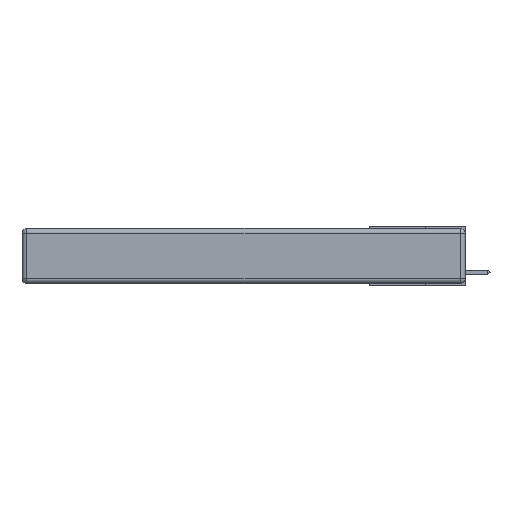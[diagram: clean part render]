
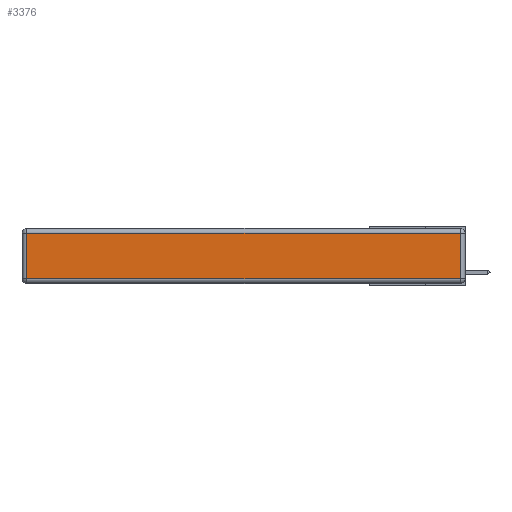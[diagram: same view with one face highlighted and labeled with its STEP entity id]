
A CAD part, left-side view. The second image highlights one B-rep face of the part: STEP entity #3376.
In plain terms, the highlighted planar face has unit normal (-1, 0, 0).
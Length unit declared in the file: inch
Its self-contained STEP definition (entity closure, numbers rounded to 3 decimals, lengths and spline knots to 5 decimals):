
#200 = CARTESIAN_POINT ( 'NONE',  ( 0., 0.03, -0.03 ) ) ;
#442 = DIRECTION ( 'NONE',  ( -1., 0., 0. ) ) ;
#705 = VECTOR ( 'NONE', #13233, 39.37008 ) ;
#1775 = EDGE_CURVE ( 'NONE', #12748, #6245, #12069, .T. ) ;
#3376 = ADVANCED_FACE ( 'NONE', ( #9781 ), #3655, .T. ) ;
#3609 = CARTESIAN_POINT ( 'NONE',  ( 0., 0., -0.343 ) ) ;
#3655 = PLANE ( 'NONE',  #8457 ) ;
#4084 = DIRECTION ( 'NONE',  ( 0., 0., -1. ) ) ;
#4110 = VERTEX_POINT ( 'NONE', #8952 ) ;
#4281 = VECTOR ( 'NONE', #13092, 39.37008 ) ;
#4509 = ORIENTED_EDGE ( 'NONE', *, *, #4553, .T. ) ;
#4553 = EDGE_CURVE ( 'NONE', #10756, #4110, #8349, .T. ) ;
#4689 = CARTESIAN_POINT ( 'NONE',  ( 0., 0.03, -0.343 ) ) ;
#5561 = EDGE_LOOP ( 'NONE', ( #4509, #13835, #14050, #12268 ) ) ;
#6245 = VERTEX_POINT ( 'NONE', #13334 ) ;
#6265 = CARTESIAN_POINT ( 'NONE',  ( 0., 2.72, -0.343 ) ) ;
#6548 = LINE ( 'NONE', #6265, #13124 ) ;
#6979 = DIRECTION ( 'NONE',  ( 0., 0., 1. ) ) ;
#7462 = VECTOR ( 'NONE', #6979, 39.37008 ) ;
#7512 = EDGE_CURVE ( 'NONE', #4110, #12748, #10045, .T. ) ;
#8291 = CARTESIAN_POINT ( 'NONE',  ( 0., 2.75, -0.03 ) ) ;
#8349 = LINE ( 'NONE', #11104, #705 ) ;
#8440 = CARTESIAN_POINT ( 'NONE',  ( 0., 2.72, -0.313 ) ) ;
#8457 = AXIS2_PLACEMENT_3D ( 'NONE', #3609, #442, #13680 ) ;
#8952 = CARTESIAN_POINT ( 'NONE',  ( 0., 0.03, -0.313 ) ) ;
#9441 = EDGE_CURVE ( 'NONE', #6245, #10756, #6548, .T. ) ;
#9781 = FACE_OUTER_BOUND ( 'NONE', #5561, .T. ) ;
#10045 = LINE ( 'NONE', #4689, #7462 ) ;
#10756 = VERTEX_POINT ( 'NONE', #8440 ) ;
#11104 = CARTESIAN_POINT ( 'NONE',  ( 0., 0., -0.313 ) ) ;
#12069 = LINE ( 'NONE', #8291, #4281 ) ;
#12268 = ORIENTED_EDGE ( 'NONE', *, *, #9441, .T. ) ;
#12748 = VERTEX_POINT ( 'NONE', #200 ) ;
#13092 = DIRECTION ( 'NONE',  ( 0., 1., 0. ) ) ;
#13124 = VECTOR ( 'NONE', #4084, 39.37008 ) ;
#13233 = DIRECTION ( 'NONE',  ( 0., -1., 0. ) ) ;
#13334 = CARTESIAN_POINT ( 'NONE',  ( 0., 2.72, -0.03 ) ) ;
#13680 = DIRECTION ( 'NONE',  ( 0., 0., 1. ) ) ;
#13835 = ORIENTED_EDGE ( 'NONE', *, *, #7512, .T. ) ;
#14050 = ORIENTED_EDGE ( 'NONE', *, *, #1775, .T. ) ;
